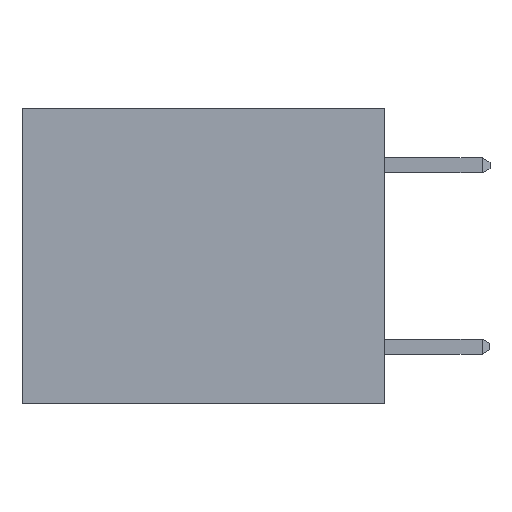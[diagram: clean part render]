
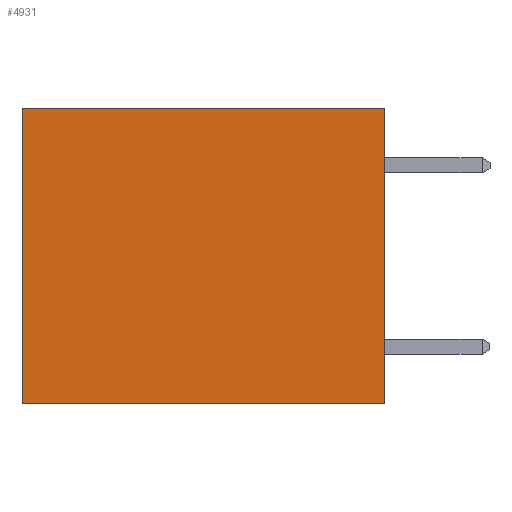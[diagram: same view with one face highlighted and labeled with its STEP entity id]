
A CAD part, left-side view. The second image highlights one B-rep face of the part: STEP entity #4931.
In plain terms, the highlighted planar face has unit normal (-1, 0, 0).
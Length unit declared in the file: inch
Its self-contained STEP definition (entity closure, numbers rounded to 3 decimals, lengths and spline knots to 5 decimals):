
#146 = ORIENTED_EDGE ( 'NONE', *, *, #2894, .T. ) ;
#557 = DIRECTION ( 'NONE',  ( 0., 0., -1. ) ) ;
#564 = EDGE_CURVE ( 'NONE', #5386, #4727, #2790, .T. ) ;
#715 = VECTOR ( 'NONE', #1693, 39.37008 ) ;
#836 = VERTEX_POINT ( 'NONE', #7751 ) ;
#1106 = ORIENTED_EDGE ( 'NONE', *, *, #3655, .F. ) ;
#1158 = DIRECTION ( 'NONE',  ( 1., 0., 0. ) ) ;
#1693 = DIRECTION ( 'NONE',  ( 0., 0., -1. ) ) ;
#2790 = LINE ( 'NONE', #2815, #715 ) ;
#2815 = CARTESIAN_POINT ( 'NONE',  ( 0.3165, 0., -0.49 ) ) ;
#2856 = VECTOR ( 'NONE', #6816, 39.37008 ) ;
#2894 = EDGE_CURVE ( 'NONE', #5474, #836, #4575, .T. ) ;
#2902 = CARTESIAN_POINT ( 'NONE',  ( 0.3165, 0.6, -0.49 ) ) ;
#3078 = EDGE_CURVE ( 'NONE', #5386, #5474, #8193, .T. ) ;
#3085 = DIRECTION ( 'NONE',  ( 0., 1., 0. ) ) ;
#3655 = EDGE_CURVE ( 'NONE', #4727, #836, #4606, .T. ) ;
#3741 = CARTESIAN_POINT ( 'NONE',  ( 0.3165, 0., 0. ) ) ;
#3848 = AXIS2_PLACEMENT_3D ( 'NONE', #4467, #1158, #557 ) ;
#4467 = CARTESIAN_POINT ( 'NONE',  ( 0.3165, 0., -0.49 ) ) ;
#4575 = LINE ( 'NONE', #2902, #2856 ) ;
#4587 = FACE_OUTER_BOUND ( 'NONE', #8146, .T. ) ;
#4606 = LINE ( 'NONE', #7359, #6524 ) ;
#4616 = ORIENTED_EDGE ( 'NONE', *, *, #3078, .T. ) ;
#4727 = VERTEX_POINT ( 'NONE', #6174 ) ;
#4867 = DIRECTION ( 'NONE',  ( 0., 1., 0. ) ) ;
#4931 = ADVANCED_FACE ( 'NONE', ( #4587 ), #7632, .F. ) ;
#5035 = ORIENTED_EDGE ( 'NONE', *, *, #564, .F. ) ;
#5386 = VERTEX_POINT ( 'NONE', #3741 ) ;
#5474 = VERTEX_POINT ( 'NONE', #5795 ) ;
#5795 = CARTESIAN_POINT ( 'NONE',  ( 0.3165, 0.6, 0. ) ) ;
#6174 = CARTESIAN_POINT ( 'NONE',  ( 0.3165, 0., -0.49 ) ) ;
#6524 = VECTOR ( 'NONE', #4867, 39.37008 ) ;
#6816 = DIRECTION ( 'NONE',  ( 0., 0., -1. ) ) ;
#7359 = CARTESIAN_POINT ( 'NONE',  ( 0.3165, 0., -0.49 ) ) ;
#7632 = PLANE ( 'NONE',  #3848 ) ;
#7751 = CARTESIAN_POINT ( 'NONE',  ( 0.3165, 0.6, -0.49 ) ) ;
#7997 = VECTOR ( 'NONE', #3085, 39.37008 ) ;
#8146 = EDGE_LOOP ( 'NONE', ( #146, #1106, #5035, #4616 ) ) ;
#8193 = LINE ( 'NONE', #8258, #7997 ) ;
#8258 = CARTESIAN_POINT ( 'NONE',  ( 0.3165, 0., 0. ) ) ;
